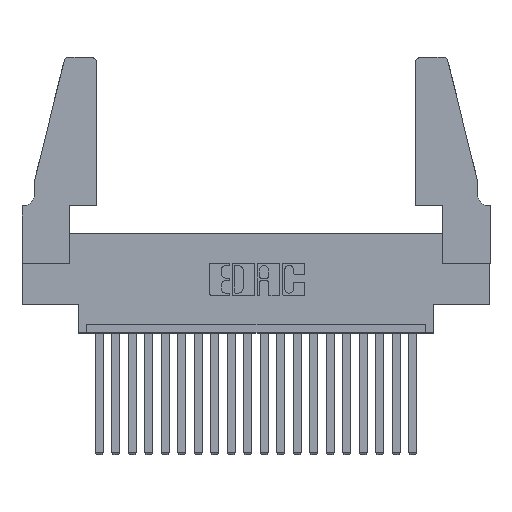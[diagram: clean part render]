
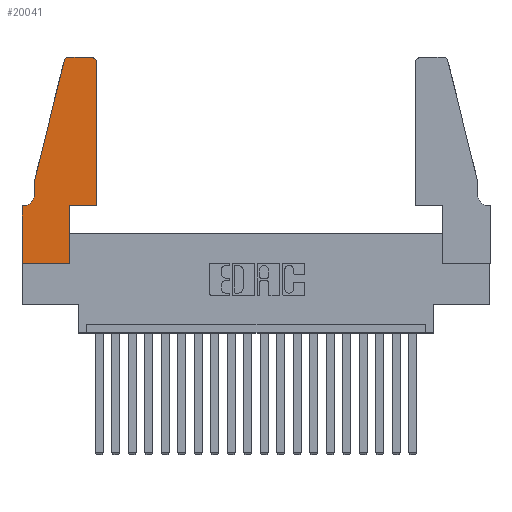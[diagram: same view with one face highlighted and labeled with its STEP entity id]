
A CAD part, top view. The second image highlights one B-rep face of the part: STEP entity #20041.
In plain terms, the highlighted planar face has unit normal (0, 0, 1).
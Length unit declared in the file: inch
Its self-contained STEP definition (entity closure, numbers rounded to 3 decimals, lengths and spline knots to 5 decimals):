
#57 = FACE_OUTER_BOUND ( 'NONE', #10056, .T. ) ;
#231 = AXIS2_PLACEMENT_3D ( 'NONE', #1783, #14238, #12724 ) ;
#460 = AXIS2_PLACEMENT_3D ( 'NONE', #19256, #19464, #7101 ) ;
#963 = VERTEX_POINT ( 'NONE', #4138 ) ;
#1057 = CARTESIAN_POINT ( 'NONE',  ( 0.2605, 1.25, 0.37 ) ) ;
#1182 = LINE ( 'NONE', #13700, #7018 ) ;
#1183 = EDGE_CURVE ( 'NONE', #15647, #17297, #11885, .T. ) ;
#1379 = LINE ( 'NONE', #6805, #18148 ) ;
#1383 = DIRECTION ( 'NONE',  ( -1., 0., 0. ) ) ;
#1408 = CARTESIAN_POINT ( 'NONE',  ( 0.284, 1.25, 0.37 ) ) ;
#1465 = AXIS2_PLACEMENT_3D ( 'NONE', #12712, #12651, #14025 ) ;
#1704 = EDGE_CURVE ( 'NONE', #963, #15647, #3307, .T. ) ;
#1740 = CARTESIAN_POINT ( 'NONE',  ( 0.4505, 1.22, 0.37 ) ) ;
#1783 = CARTESIAN_POINT ( 'NONE',  ( 0.4205, 1.22, 0.37 ) ) ;
#2041 = ORIENTED_EDGE ( 'NONE', *, *, #19594, .T. ) ;
#2061 = CARTESIAN_POINT ( 'NONE',  ( 0.25487, 1.22718, 0.37 ) ) ;
#2333 = CIRCLE ( 'NONE', #231, 0.03 ) ;
#2367 = DIRECTION ( 'NONE',  ( 0., -1., 0. ) ) ;
#2465 = CARTESIAN_POINT ( 'NONE',  ( 0.284, 1.22, 0.37 ) ) ;
#2866 = CARTESIAN_POINT ( 'NONE',  ( 0.0055, 0.35, 0.37 ) ) ;
#3002 = EDGE_CURVE ( 'NONE', #7501, #963, #1379, .T. ) ;
#3307 = LINE ( 'NONE', #4788, #12595 ) ;
#3719 = LINE ( 'NONE', #10301, #17104 ) ;
#3956 = VERTEX_POINT ( 'NONE', #6593 ) ;
#4115 = DIRECTION ( 'NONE',  ( 0., 1., 0. ) ) ;
#4138 = CARTESIAN_POINT ( 'NONE',  ( 0.0755, 0.5, 0.37 ) ) ;
#4233 = AXIS2_PLACEMENT_3D ( 'NONE', #2465, #11897, #13794 ) ;
#4788 = CARTESIAN_POINT ( 'NONE',  ( 0.0755, 0.5, 0.37 ) ) ;
#5031 = VECTOR ( 'NONE', #7450, 39.37008 ) ;
#5662 = LINE ( 'NONE', #5831, #15175 ) ;
#5831 = CARTESIAN_POINT ( 'NONE',  ( 0., 0., 0.37 ) ) ;
#6593 = CARTESIAN_POINT ( 'NONE',  ( 0., 0., 0.37 ) ) ;
#6612 = ORIENTED_EDGE ( 'NONE', *, *, #3002, .T. ) ;
#6734 = DIRECTION ( 'NONE',  ( -0.239, -0.971, 0. ) ) ;
#6805 = CARTESIAN_POINT ( 'NONE',  ( 0.0755, 0.5, 0.37 ) ) ;
#6866 = CARTESIAN_POINT ( 'NONE',  ( 0.4505, 0.35, 0.37 ) ) ;
#6916 = DIRECTION ( 'NONE',  ( 1., 0., 0. ) ) ;
#6964 = CARTESIAN_POINT ( 'NONE',  ( 0., 0.35, 0.37 ) ) ;
#6994 = EDGE_CURVE ( 'NONE', #10909, #7621, #11739, .T. ) ;
#7018 = VECTOR ( 'NONE', #1383, 39.37008 ) ;
#7101 = DIRECTION ( 'NONE',  ( -1., 0., 0. ) ) ;
#7450 = DIRECTION ( 'NONE',  ( -1., 0., 0. ) ) ;
#7501 = VERTEX_POINT ( 'NONE', #2061 ) ;
#7621 = VERTEX_POINT ( 'NONE', #1740 ) ;
#8074 = ORIENTED_EDGE ( 'NONE', *, *, #15353, .T. ) ;
#8331 = ORIENTED_EDGE ( 'NONE', *, *, #15964, .T. ) ;
#8672 = LINE ( 'NONE', #1057, #5031 ) ;
#9445 = EDGE_CURVE ( 'NONE', #16047, #3956, #14814, .T. ) ;
#9613 = CARTESIAN_POINT ( 'NONE',  ( 0.4505, 0.35, 0.37 ) ) ;
#9797 = EDGE_CURVE ( 'NONE', #17297, #16047, #1182, .T. ) ;
#10056 = EDGE_LOOP ( 'NONE', ( #8074, #12682, #6612, #14554, #10427, #13283, #19854, #19571, #13020, #2041, #15866, #8331 ) ) ;
#10301 = CARTESIAN_POINT ( 'NONE',  ( 0.2865, 0.35, 0.37 ) ) ;
#10427 = ORIENTED_EDGE ( 'NONE', *, *, #1183, .T. ) ;
#10860 = DIRECTION ( 'NONE',  ( 0., -1., 0. ) ) ;
#10909 = VERTEX_POINT ( 'NONE', #9613 ) ;
#11479 = CARTESIAN_POINT ( 'NONE',  ( 0.2865, 0., 0.37 ) ) ;
#11739 = LINE ( 'NONE', #6866, #15868 ) ;
#11885 = CIRCLE ( 'NONE', #460, 0.07 ) ;
#11897 = DIRECTION ( 'NONE',  ( 0., 0., 1. ) ) ;
#12275 = CARTESIAN_POINT ( 'NONE',  ( 0.4205, 1.25, 0.37 ) ) ;
#12595 = VECTOR ( 'NONE', #10860, 39.37008 ) ;
#12651 = DIRECTION ( 'NONE',  ( 0., 0., 1. ) ) ;
#12682 = ORIENTED_EDGE ( 'NONE', *, *, #14639, .T. ) ;
#12712 = CARTESIAN_POINT ( 'NONE',  ( 0., 0.35, 0.37 ) ) ;
#12724 = DIRECTION ( 'NONE',  ( 1., 0., 0. ) ) ;
#12834 = DIRECTION ( 'NONE',  ( 0., 1., 0. ) ) ;
#13020 = ORIENTED_EDGE ( 'NONE', *, *, #19059, .T. ) ;
#13278 = CARTESIAN_POINT ( 'NONE',  ( 0.4505, 0.35, 0.37 ) ) ;
#13283 = ORIENTED_EDGE ( 'NONE', *, *, #9797, .T. ) ;
#13700 = CARTESIAN_POINT ( 'NONE',  ( 0.0755, 0.35, 0.37 ) ) ;
#13794 = DIRECTION ( 'NONE',  ( 1., 0., 0. ) ) ;
#13878 = CARTESIAN_POINT ( 'NONE',  ( 0.2865, 0.35, 0.37 ) ) ;
#14025 = DIRECTION ( 'NONE',  ( 1., 0., 0. ) ) ;
#14238 = DIRECTION ( 'NONE',  ( 0., 0., 1. ) ) ;
#14412 = CARTESIAN_POINT ( 'NONE',  ( 0.0755, 0.42, 0.37 ) ) ;
#14554 = ORIENTED_EDGE ( 'NONE', *, *, #1704, .T. ) ;
#14639 = EDGE_CURVE ( 'NONE', #15824, #7501, #14795, .T. ) ;
#14795 = CIRCLE ( 'NONE', #4233, 0.03 ) ;
#14814 = LINE ( 'NONE', #16391, #20144 ) ;
#15175 = VECTOR ( 'NONE', #16691, 39.37008 ) ;
#15353 = EDGE_CURVE ( 'NONE', #15521, #15824, #8672, .T. ) ;
#15521 = VERTEX_POINT ( 'NONE', #12275 ) ;
#15647 = VERTEX_POINT ( 'NONE', #14412 ) ;
#15824 = VERTEX_POINT ( 'NONE', #1408 ) ;
#15866 = ORIENTED_EDGE ( 'NONE', *, *, #6994, .T. ) ;
#15868 = VECTOR ( 'NONE', #12834, 39.37008 ) ;
#15964 = EDGE_CURVE ( 'NONE', #7621, #15521, #2333, .T. ) ;
#16047 = VERTEX_POINT ( 'NONE', #6964 ) ;
#16367 = VERTEX_POINT ( 'NONE', #11479 ) ;
#16391 = CARTESIAN_POINT ( 'NONE',  ( 0., 0., 0.37 ) ) ;
#16691 = DIRECTION ( 'NONE',  ( 1., 0., 0. ) ) ;
#17082 = VECTOR ( 'NONE', #6916, 39.37008 ) ;
#17104 = VECTOR ( 'NONE', #4115, 39.37008 ) ;
#17297 = VERTEX_POINT ( 'NONE', #2866 ) ;
#17396 = PLANE ( 'NONE',  #1465 ) ;
#18148 = VECTOR ( 'NONE', #6734, 39.37008 ) ;
#18302 = LINE ( 'NONE', #13278, #17082 ) ;
#18591 = VERTEX_POINT ( 'NONE', #13878 ) ;
#19059 = EDGE_CURVE ( 'NONE', #16367, #18591, #3719, .T. ) ;
#19235 = EDGE_CURVE ( 'NONE', #3956, #16367, #5662, .T. ) ;
#19256 = CARTESIAN_POINT ( 'NONE',  ( 0.0055, 0.42, 0.37 ) ) ;
#19464 = DIRECTION ( 'NONE',  ( 0., 0., -1. ) ) ;
#19571 = ORIENTED_EDGE ( 'NONE', *, *, #19235, .T. ) ;
#19594 = EDGE_CURVE ( 'NONE', #18591, #10909, #18302, .T. ) ;
#19854 = ORIENTED_EDGE ( 'NONE', *, *, #9445, .T. ) ;
#20041 = ADVANCED_FACE ( 'NONE', ( #57 ), #17396, .T. ) ;
#20144 = VECTOR ( 'NONE', #2367, 39.37008 ) ;
